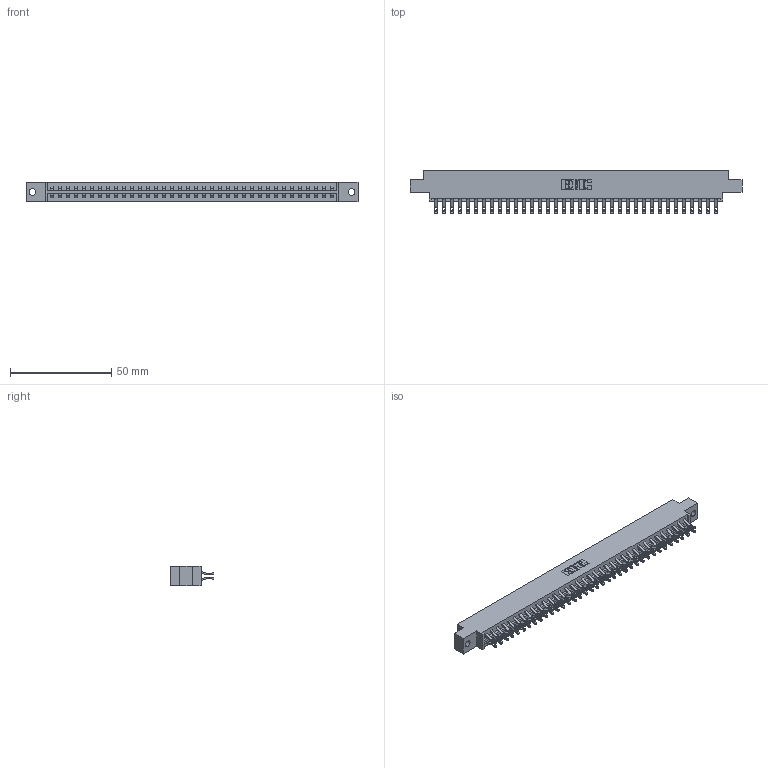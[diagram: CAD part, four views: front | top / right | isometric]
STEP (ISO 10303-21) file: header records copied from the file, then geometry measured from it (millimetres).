
FILE_DESCRIPTION (( 'STEP AP203' ), '1' );
FILE_NAME ('833-072-555-802.STEP', '2020-06-05T14:45:31', ( '' ), ( '' ), 'SwSTEP 2.0', 'SolidWorks 2020', '' );
FILE_SCHEMA (( 'CONFIG_CONTROL_DESIGN' ));
Length unit declared in the file: inch
Products named in the file (3): 345-292-001_555 Tail; 833 Part_Offset - .128 Dia; 833-072-555-802
Assembly tree (73 placements, depth 2):
  833-072-555-802
    833 Part_Offset - .128 Dia
    345-292-001_555 Tail  x72
Bounding box: 164.19 x 21.47 x 9.4 mm (x, y, z)
Volume: 16650.7 mm3; surface area: 20349.3 mm2
Topology: 73 solids, 73 shells, 4294 faces, 13499 edges, 8998 vertices
Faces by surface type: plane 2522, cylinder 1772
Entity records: 24397 total; most frequent: CARTESIAN_POINT 4088, ORIENTED_EDGE 3994, DIRECTION 3473, EDGE_CURVE 1997, LINE 1849, VECTOR 1849, VERTEX_POINT 1330, AXIS2_PLACEMENT_3D 812
